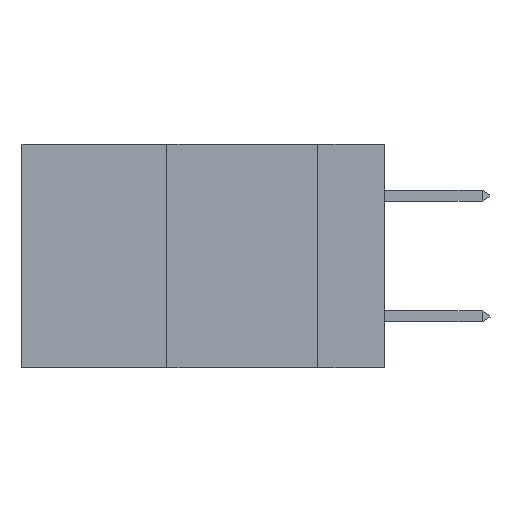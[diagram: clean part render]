
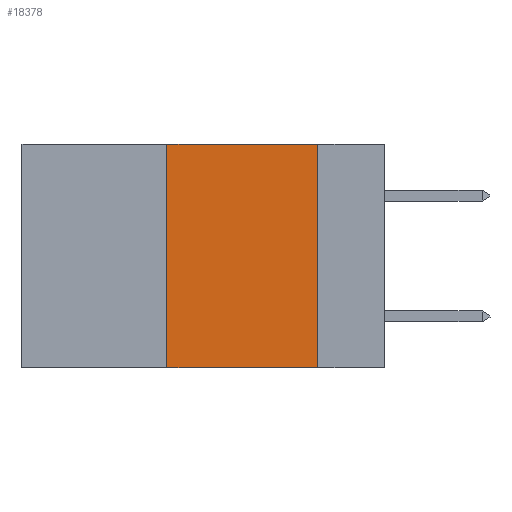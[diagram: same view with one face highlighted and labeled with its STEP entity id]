
A CAD part, left-side view. The second image highlights one B-rep face of the part: STEP entity #18378.
In plain terms, the highlighted planar face has unit normal (-1, 0, 0).
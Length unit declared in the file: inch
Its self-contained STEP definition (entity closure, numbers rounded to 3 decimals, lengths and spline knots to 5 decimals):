
#807 = CARTESIAN_POINT ( 'NONE',  ( 0., 0.36, 0. ) ) ;
#932 = LINE ( 'NONE', #22135, #18470 ) ;
#1193 = DIRECTION ( 'NONE',  ( 0., 0., -1. ) ) ;
#4994 = FACE_OUTER_BOUND ( 'NONE', #7492, .T. ) ;
#5485 = CARTESIAN_POINT ( 'NONE',  ( 0., 0.6, -0.37 ) ) ;
#7068 = ORIENTED_EDGE ( 'NONE', *, *, #14077, .F. ) ;
#7344 = EDGE_CURVE ( 'NONE', #15111, #7402, #932, .T. ) ;
#7402 = VERTEX_POINT ( 'NONE', #22201 ) ;
#7492 = EDGE_LOOP ( 'NONE', ( #15126, #7068, #16215, #20804 ) ) ;
#7819 = VECTOR ( 'NONE', #21101, 39.37008 ) ;
#8150 = CARTESIAN_POINT ( 'NONE',  ( 0., 0.11, 0. ) ) ;
#8665 = DIRECTION ( 'NONE',  ( 0., -1., 0. ) ) ;
#8952 = CARTESIAN_POINT ( 'NONE',  ( 0., 0.6, 0. ) ) ;
#10220 = CARTESIAN_POINT ( 'NONE',  ( 0., 0.36, 0. ) ) ;
#10651 = DIRECTION ( 'NONE',  ( 0., 0., -1. ) ) ;
#12751 = VERTEX_POINT ( 'NONE', #17246 ) ;
#13265 = LINE ( 'NONE', #10220, #20828 ) ;
#13885 = VECTOR ( 'NONE', #8665, 39.37008 ) ;
#14077 = EDGE_CURVE ( 'NONE', #18085, #15111, #19009, .T. ) ;
#15111 = VERTEX_POINT ( 'NONE', #8150 ) ;
#15126 = ORIENTED_EDGE ( 'NONE', *, *, #7344, .F. ) ;
#15852 = EDGE_CURVE ( 'NONE', #12751, #18085, #13265, .T. ) ;
#16215 = ORIENTED_EDGE ( 'NONE', *, *, #15852, .F. ) ;
#17246 = CARTESIAN_POINT ( 'NONE',  ( 0., 0.36, -0.37 ) ) ;
#17512 = LINE ( 'NONE', #5485, #7819 ) ;
#17857 = EDGE_CURVE ( 'NONE', #12751, #7402, #17512, .T. ) ;
#18085 = VERTEX_POINT ( 'NONE', #807 ) ;
#18378 = ADVANCED_FACE ( 'NONE', ( #4994 ), #19175, .F. ) ;
#18470 = VECTOR ( 'NONE', #1193, 39.37008 ) ;
#18814 = DIRECTION ( 'NONE',  ( 0., 0., 1. ) ) ;
#18902 = AXIS2_PLACEMENT_3D ( 'NONE', #8952, #20920, #10651 ) ;
#19009 = LINE ( 'NONE', #20665, #13885 ) ;
#19175 = PLANE ( 'NONE',  #18902 ) ;
#20665 = CARTESIAN_POINT ( 'NONE',  ( 0., 0.6, 0. ) ) ;
#20804 = ORIENTED_EDGE ( 'NONE', *, *, #17857, .T. ) ;
#20828 = VECTOR ( 'NONE', #18814, 39.37008 ) ;
#20920 = DIRECTION ( 'NONE',  ( 1., 0., 0. ) ) ;
#21101 = DIRECTION ( 'NONE',  ( 0., -1., 0. ) ) ;
#22135 = CARTESIAN_POINT ( 'NONE',  ( 0., 0.11, 0. ) ) ;
#22201 = CARTESIAN_POINT ( 'NONE',  ( 0., 0.11, -0.37 ) ) ;
